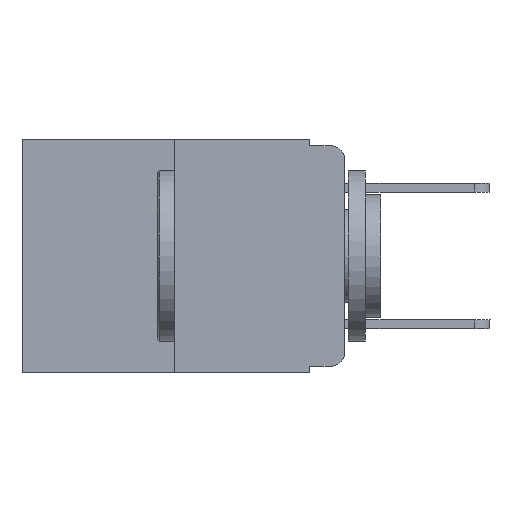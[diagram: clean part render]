
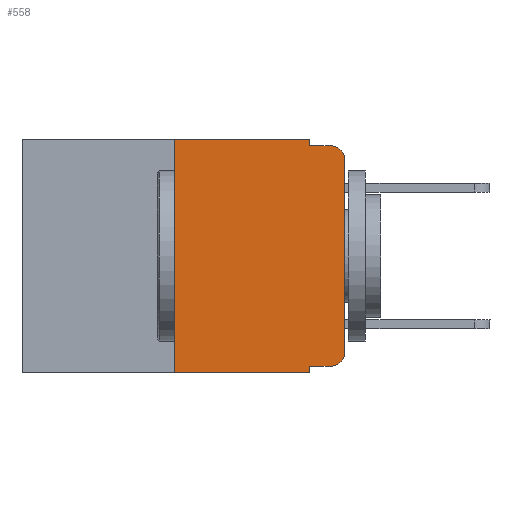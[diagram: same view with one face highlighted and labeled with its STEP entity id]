
A CAD part, left-side view. The second image highlights one B-rep face of the part: STEP entity #558.
In plain terms, the highlighted planar face has unit normal (-1, 0, 0).
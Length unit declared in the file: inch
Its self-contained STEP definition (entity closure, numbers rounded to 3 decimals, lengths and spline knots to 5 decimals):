
#117 = ORIENTED_EDGE ( 'NONE', *, *, #10061, .F. ) ;
#251 = VERTEX_POINT ( 'NONE', #13639 ) ;
#497 = CIRCLE ( 'NONE', #4140, 0.02 ) ;
#558 = ADVANCED_FACE ( 'NONE', ( #11415 ), #17839, .F. ) ;
#1147 = DIRECTION ( 'NONE',  ( 0., -1., 0. ) ) ;
#1509 = CARTESIAN_POINT ( 'NONE',  ( 0., 0.051, 0. ) ) ;
#1522 = CARTESIAN_POINT ( 'NONE',  ( 0., 0.473, -0.343 ) ) ;
#1529 = DIRECTION ( 'NONE',  ( -1., 0., 0. ) ) ;
#1581 = CARTESIAN_POINT ( 'NONE',  ( 0., 0.25, 0. ) ) ;
#1704 = CARTESIAN_POINT ( 'NONE',  ( 0., 0.051, -0.01 ) ) ;
#1854 = CARTESIAN_POINT ( 'NONE',  ( 0., 0.051, -0.343 ) ) ;
#2259 = VECTOR ( 'NONE', #15736, 39.37008 ) ;
#2855 = VERTEX_POINT ( 'NONE', #1854 ) ;
#2901 = LINE ( 'NONE', #9314, #2259 ) ;
#3058 = CARTESIAN_POINT ( 'NONE',  ( 0., 0.02, -0.01 ) ) ;
#3169 = DIRECTION ( 'NONE',  ( 0., 0., -1. ) ) ;
#3211 = EDGE_CURVE ( 'NONE', #17042, #251, #8322, .T. ) ;
#3289 = DIRECTION ( 'NONE',  ( 0., 0., -1. ) ) ;
#3404 = VECTOR ( 'NONE', #5277, 39.37008 ) ;
#3464 = LINE ( 'NONE', #3663, #14649 ) ;
#3663 = CARTESIAN_POINT ( 'NONE',  ( 0., 0.051, -0.333 ) ) ;
#3730 = ORIENTED_EDGE ( 'NONE', *, *, #17402, .F. ) ;
#4140 = AXIS2_PLACEMENT_3D ( 'NONE', #17861, #13014, #19435 ) ;
#4152 = DIRECTION ( 'NONE',  ( 0., 0., -1. ) ) ;
#4269 = EDGE_CURVE ( 'NONE', #15528, #10873, #8995, .T. ) ;
#4550 = VERTEX_POINT ( 'NONE', #13329 ) ;
#4604 = ORIENTED_EDGE ( 'NONE', *, *, #7071, .T. ) ;
#4744 = LINE ( 'NONE', #1522, #19872 ) ;
#5277 = DIRECTION ( 'NONE',  ( 0., 0., 1. ) ) ;
#5302 = EDGE_CURVE ( 'NONE', #14204, #15528, #7770, .T. ) ;
#5363 = VERTEX_POINT ( 'NONE', #10002 ) ;
#5371 = DIRECTION ( 'NONE',  ( 0., 0., -1. ) ) ;
#5615 = ORIENTED_EDGE ( 'NONE', *, *, #16334, .T. ) ;
#5617 = EDGE_CURVE ( 'NONE', #251, #10873, #497, .T. ) ;
#6283 = VECTOR ( 'NONE', #1147, 39.37008 ) ;
#7071 = EDGE_CURVE ( 'NONE', #17466, #4550, #3464, .T. ) ;
#7248 = AXIS2_PLACEMENT_3D ( 'NONE', #20668, #1529, #3289 ) ;
#7628 = DIRECTION ( 'NONE',  ( 0., 0., 1. ) ) ;
#7770 = LINE ( 'NONE', #1509, #16923 ) ;
#8277 = CIRCLE ( 'NONE', #7248, 0.02 ) ;
#8322 = LINE ( 'NONE', #9713, #3404 ) ;
#8364 = CARTESIAN_POINT ( 'NONE',  ( 0., 0.051, 0. ) ) ;
#8681 = LINE ( 'NONE', #8898, #9080 ) ;
#8898 = CARTESIAN_POINT ( 'NONE',  ( 0., 0.051, 0. ) ) ;
#8995 = LINE ( 'NONE', #17027, #6283 ) ;
#9080 = VECTOR ( 'NONE', #4152, 39.37008 ) ;
#9314 = CARTESIAN_POINT ( 'NONE',  ( 0., 0.473, 0. ) ) ;
#9713 = CARTESIAN_POINT ( 'NONE',  ( 0., 0., 0. ) ) ;
#10002 = CARTESIAN_POINT ( 'NONE',  ( 0., 0.25, -0.343 ) ) ;
#10061 = EDGE_CURVE ( 'NONE', #16805, #14204, #2901, .T. ) ;
#10595 = EDGE_CURVE ( 'NONE', #4550, #17042, #8277, .T. ) ;
#10873 = VERTEX_POINT ( 'NONE', #3058 ) ;
#11415 = FACE_OUTER_BOUND ( 'NONE', #16236, .T. ) ;
#12398 = VECTOR ( 'NONE', #7628, 39.37008 ) ;
#13014 = DIRECTION ( 'NONE',  ( -1., 0., 0. ) ) ;
#13102 = CARTESIAN_POINT ( 'NONE',  ( 0., 0.473, 0. ) ) ;
#13329 = CARTESIAN_POINT ( 'NONE',  ( 0., 0.02, -0.333 ) ) ;
#13639 = CARTESIAN_POINT ( 'NONE',  ( 0., 0., -0.03 ) ) ;
#14054 = ORIENTED_EDGE ( 'NONE', *, *, #19024, .F. ) ;
#14204 = VERTEX_POINT ( 'NONE', #8364 ) ;
#14526 = CARTESIAN_POINT ( 'NONE',  ( 0., 0., -0.313 ) ) ;
#14649 = VECTOR ( 'NONE', #18093, 39.37008 ) ;
#14842 = ORIENTED_EDGE ( 'NONE', *, *, #10595, .T. ) ;
#15528 = VERTEX_POINT ( 'NONE', #1704 ) ;
#15736 = DIRECTION ( 'NONE',  ( 0., -1., 0. ) ) ;
#15764 = CARTESIAN_POINT ( 'NONE',  ( 0., 0.051, -0.333 ) ) ;
#15957 = CARTESIAN_POINT ( 'NONE',  ( 0., 0.25, 0. ) ) ;
#15980 = LINE ( 'NONE', #1581, #12398 ) ;
#16160 = ORIENTED_EDGE ( 'NONE', *, *, #5617, .T. ) ;
#16236 = EDGE_LOOP ( 'NONE', ( #19575, #16160, #19013, #18893, #117, #3730, #5615, #14054, #4604, #14842 ) ) ;
#16289 = AXIS2_PLACEMENT_3D ( 'NONE', #13102, #19529, #5371 ) ;
#16334 = EDGE_CURVE ( 'NONE', #5363, #2855, #4744, .T. ) ;
#16805 = VERTEX_POINT ( 'NONE', #15957 ) ;
#16923 = VECTOR ( 'NONE', #3169, 39.37008 ) ;
#17027 = CARTESIAN_POINT ( 'NONE',  ( 0., 0.051, -0.01 ) ) ;
#17042 = VERTEX_POINT ( 'NONE', #14526 ) ;
#17402 = EDGE_CURVE ( 'NONE', #5363, #16805, #15980, .T. ) ;
#17466 = VERTEX_POINT ( 'NONE', #15764 ) ;
#17839 = PLANE ( 'NONE',  #16289 ) ;
#17861 = CARTESIAN_POINT ( 'NONE',  ( 0., 0.02, -0.03 ) ) ;
#18093 = DIRECTION ( 'NONE',  ( 0., -1., 0. ) ) ;
#18893 = ORIENTED_EDGE ( 'NONE', *, *, #5302, .F. ) ;
#19013 = ORIENTED_EDGE ( 'NONE', *, *, #4269, .F. ) ;
#19024 = EDGE_CURVE ( 'NONE', #17466, #2855, #8681, .T. ) ;
#19435 = DIRECTION ( 'NONE',  ( 0., 0., -1. ) ) ;
#19529 = DIRECTION ( 'NONE',  ( 1., 0., 0. ) ) ;
#19575 = ORIENTED_EDGE ( 'NONE', *, *, #3211, .T. ) ;
#19872 = VECTOR ( 'NONE', #20447, 39.37008 ) ;
#20447 = DIRECTION ( 'NONE',  ( 0., -1., 0. ) ) ;
#20668 = CARTESIAN_POINT ( 'NONE',  ( 0., 0.02, -0.313 ) ) ;
